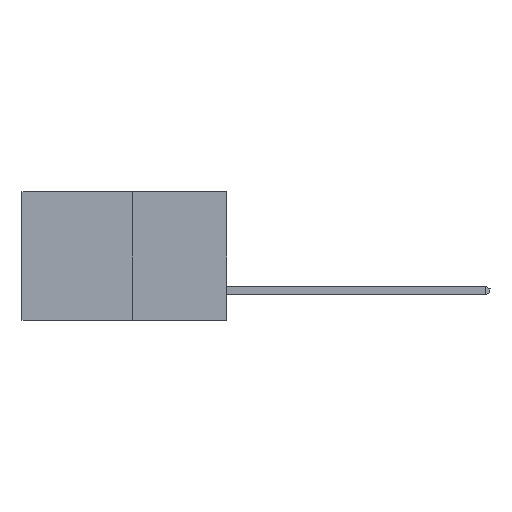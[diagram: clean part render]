
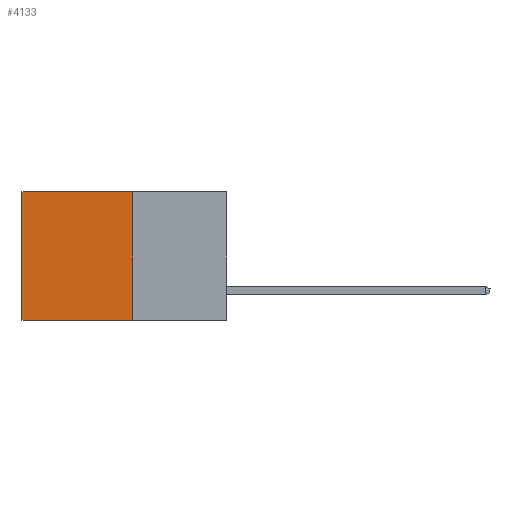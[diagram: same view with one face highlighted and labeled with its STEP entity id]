
A CAD part, left-side view. The second image highlights one B-rep face of the part: STEP entity #4133.
In plain terms, the highlighted planar face has unit normal (-1, 0, 0).
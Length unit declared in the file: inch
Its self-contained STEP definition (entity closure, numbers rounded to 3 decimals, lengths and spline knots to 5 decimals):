
#563 = LINE ( 'NONE', #2726, #10567 ) ;
#872 = AXIS2_PLACEMENT_3D ( 'NONE', #1458, #9891, #9869 ) ;
#888 = DIRECTION ( 'NONE',  ( 0., 0., -1. ) ) ;
#1256 = VERTEX_POINT ( 'NONE', #7737 ) ;
#1458 = CARTESIAN_POINT ( 'NONE',  ( 0.277, 0.27, -0.37 ) ) ;
#1670 = LINE ( 'NONE', #6355, #9624 ) ;
#1908 = VERTEX_POINT ( 'NONE', #9230 ) ;
#2141 = ORIENTED_EDGE ( 'NONE', *, *, #6010, .T. ) ;
#2346 = ORIENTED_EDGE ( 'NONE', *, *, #10636, .F. ) ;
#2364 = ORIENTED_EDGE ( 'NONE', *, *, #3873, .F. ) ;
#2565 = VERTEX_POINT ( 'NONE', #7462 ) ;
#2726 = CARTESIAN_POINT ( 'NONE',  ( 0.277, 0.59, -0.37 ) ) ;
#2840 = ORIENTED_EDGE ( 'NONE', *, *, #3125, .T. ) ;
#3125 = EDGE_CURVE ( 'NONE', #13077, #2565, #1670, .T. ) ;
#3822 = FACE_OUTER_BOUND ( 'NONE', #5466, .T. ) ;
#3873 = EDGE_CURVE ( 'NONE', #13077, #1908, #8828, .T. ) ;
#4003 = VECTOR ( 'NONE', #888, 39.37008 ) ;
#4133 = ADVANCED_FACE ( 'NONE', ( #3822 ), #7863, .F. ) ;
#5466 = EDGE_LOOP ( 'NONE', ( #2141, #2346, #2364, #2840 ) ) ;
#5927 = CARTESIAN_POINT ( 'NONE',  ( 0.277, 0.27, -0.37 ) ) ;
#6010 = EDGE_CURVE ( 'NONE', #2565, #1256, #563, .T. ) ;
#6155 = LINE ( 'NONE', #5927, #8869 ) ;
#6355 = CARTESIAN_POINT ( 'NONE',  ( 0.277, 0.27, 0. ) ) ;
#7462 = CARTESIAN_POINT ( 'NONE',  ( 0.277, 0.59, 0. ) ) ;
#7737 = CARTESIAN_POINT ( 'NONE',  ( 0.277, 0.59, -0.37 ) ) ;
#7863 = PLANE ( 'NONE',  #872 ) ;
#8828 = LINE ( 'NONE', #13179, #4003 ) ;
#8869 = VECTOR ( 'NONE', #12910, 39.37008 ) ;
#8905 = CARTESIAN_POINT ( 'NONE',  ( 0.277, 0.27, 0. ) ) ;
#9230 = CARTESIAN_POINT ( 'NONE',  ( 0.277, 0.27, -0.37 ) ) ;
#9624 = VECTOR ( 'NONE', #13059, 39.37008 ) ;
#9869 = DIRECTION ( 'NONE',  ( 0., 0., -1. ) ) ;
#9891 = DIRECTION ( 'NONE',  ( 1., 0., 0. ) ) ;
#10567 = VECTOR ( 'NONE', #11900, 39.37008 ) ;
#10636 = EDGE_CURVE ( 'NONE', #1908, #1256, #6155, .T. ) ;
#11900 = DIRECTION ( 'NONE',  ( 0., 0., -1. ) ) ;
#12910 = DIRECTION ( 'NONE',  ( 0., 1., 0. ) ) ;
#13059 = DIRECTION ( 'NONE',  ( 0., 1., 0. ) ) ;
#13077 = VERTEX_POINT ( 'NONE', #8905 ) ;
#13179 = CARTESIAN_POINT ( 'NONE',  ( 0.277, 0.27, -0.37 ) ) ;
